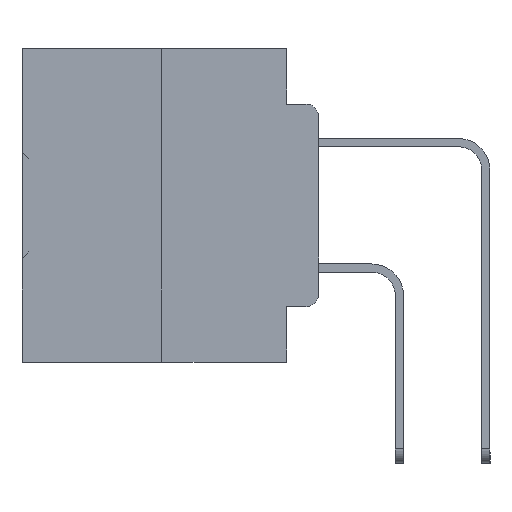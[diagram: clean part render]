
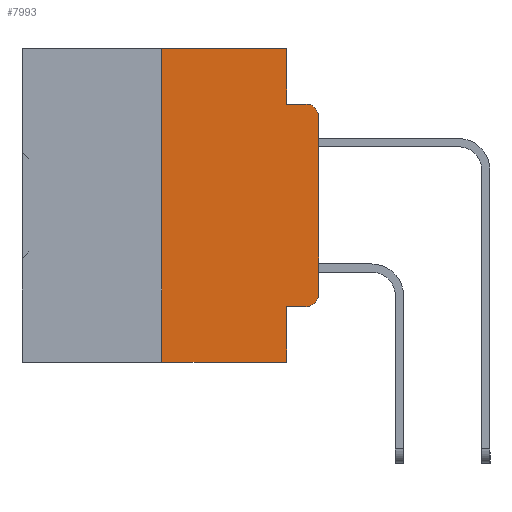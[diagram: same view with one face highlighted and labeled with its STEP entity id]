
A CAD part, left-side view. The second image highlights one B-rep face of the part: STEP entity #7993.
In plain terms, the highlighted planar face has unit normal (-1, 0, 0).
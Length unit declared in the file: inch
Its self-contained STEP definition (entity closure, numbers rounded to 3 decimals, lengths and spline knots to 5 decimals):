
#244 = EDGE_CURVE ( 'NONE', #16485, #21619, #24784, .T. ) ;
#370 = AXIS2_PLACEMENT_3D ( 'NONE', #22116, #3656, #25164 ) ;
#1568 = CARTESIAN_POINT ( 'NONE',  ( 0., 0.051, -0.4115 ) ) ;
#2293 = EDGE_CURVE ( 'NONE', #29441, #16485, #23737, .T. ) ;
#2381 = CARTESIAN_POINT ( 'NONE',  ( 0., 0.02, -0.0885 ) ) ;
#2928 = ORIENTED_EDGE ( 'NONE', *, *, #25778, .F. ) ;
#3067 = CARTESIAN_POINT ( 'NONE',  ( 0., 0.051, 0. ) ) ;
#3404 = ORIENTED_EDGE ( 'NONE', *, *, #37893, .F. ) ;
#3656 = DIRECTION ( 'NONE',  ( -1., 0., 0. ) ) ;
#4323 = ORIENTED_EDGE ( 'NONE', *, *, #13835, .T. ) ;
#5776 = CARTESIAN_POINT ( 'NONE',  ( 0., 0.473, 0. ) ) ;
#6856 = LINE ( 'NONE', #16288, #30311 ) ;
#6938 = CARTESIAN_POINT ( 'NONE',  ( 0., 0.051, -0.0885 ) ) ;
#7919 = CARTESIAN_POINT ( 'NONE',  ( 0., 0.473, 0. ) ) ;
#7993 = ADVANCED_FACE ( 'NONE', ( #14914 ), #30257, .F. ) ;
#8205 = VECTOR ( 'NONE', #10116, 39.37008 ) ;
#8875 = LINE ( 'NONE', #24295, #37418 ) ;
#8999 = DIRECTION ( 'NONE',  ( 0., -1., 0. ) ) ;
#9776 = EDGE_CURVE ( 'NONE', #32837, #11444, #29019, .T. ) ;
#10037 = LINE ( 'NONE', #13108, #33409 ) ;
#10041 = DIRECTION ( 'NONE',  ( 0., 0., -1. ) ) ;
#10116 = DIRECTION ( 'NONE',  ( 0., 0., -1. ) ) ;
#10364 = VERTEX_POINT ( 'NONE', #23327 ) ;
#10678 = CIRCLE ( 'NONE', #370, 0.02 ) ;
#10731 = CARTESIAN_POINT ( 'NONE',  ( 0., 0.02, -0.1085 ) ) ;
#11444 = VERTEX_POINT ( 'NONE', #3067 ) ;
#13108 = CARTESIAN_POINT ( 'NONE',  ( 0., 0.25, 0. ) ) ;
#13145 = ORIENTED_EDGE ( 'NONE', *, *, #17663, .T. ) ;
#13481 = DIRECTION ( 'NONE',  ( 0., 0., 1. ) ) ;
#13612 = ORIENTED_EDGE ( 'NONE', *, *, #9776, .F. ) ;
#13835 = EDGE_CURVE ( 'NONE', #10364, #39304, #8875, .T. ) ;
#13854 = LINE ( 'NONE', #16884, #38030 ) ;
#14914 = FACE_OUTER_BOUND ( 'NONE', #22867, .T. ) ;
#15589 = EDGE_CURVE ( 'NONE', #24892, #29441, #10678, .T. ) ;
#16228 = CARTESIAN_POINT ( 'NONE',  ( 0., 0.051, -0.4115 ) ) ;
#16288 = CARTESIAN_POINT ( 'NONE',  ( 0., 0.051, 0. ) ) ;
#16485 = VERTEX_POINT ( 'NONE', #23121 ) ;
#16884 = CARTESIAN_POINT ( 'NONE',  ( 0., 0.051, -0.0885 ) ) ;
#17663 = EDGE_CURVE ( 'NONE', #33151, #24892, #30477, .T. ) ;
#18224 = DIRECTION ( 'NONE',  ( 0., 0., -1. ) ) ;
#18932 = ORIENTED_EDGE ( 'NONE', *, *, #244, .T. ) ;
#20579 = CARTESIAN_POINT ( 'NONE',  ( 0., 0., -0.3915 ) ) ;
#20814 = ORIENTED_EDGE ( 'NONE', *, *, #29831, .F. ) ;
#20932 = CARTESIAN_POINT ( 'NONE',  ( 0., 0.051, -0.5 ) ) ;
#21330 = VERTEX_POINT ( 'NONE', #6938 ) ;
#21619 = VERTEX_POINT ( 'NONE', #2381 ) ;
#21739 = ORIENTED_EDGE ( 'NONE', *, *, #27785, .F. ) ;
#22116 = CARTESIAN_POINT ( 'NONE',  ( 0., 0.02, -0.3915 ) ) ;
#22867 = EDGE_LOOP ( 'NONE', ( #26009, #18932, #3404, #20814, #13612, #21739, #4323, #2928, #13145, #37335 ) ) ;
#22903 = VECTOR ( 'NONE', #29284, 39.37008 ) ;
#23121 = CARTESIAN_POINT ( 'NONE',  ( 0., 0., -0.1085 ) ) ;
#23327 = CARTESIAN_POINT ( 'NONE',  ( 0., 0.25, -0.5 ) ) ;
#23385 = VECTOR ( 'NONE', #37358, 39.37008 ) ;
#23723 = AXIS2_PLACEMENT_3D ( 'NONE', #5776, #36305, #18224 ) ;
#23737 = LINE ( 'NONE', #31703, #30823 ) ;
#24295 = CARTESIAN_POINT ( 'NONE',  ( 0., 0.473, -0.5 ) ) ;
#24784 = CIRCLE ( 'NONE', #30597, 0.02 ) ;
#24892 = VERTEX_POINT ( 'NONE', #27155 ) ;
#25164 = DIRECTION ( 'NONE',  ( 0., 0., -1. ) ) ;
#25706 = DIRECTION ( 'NONE',  ( 0., 0., -1. ) ) ;
#25778 = EDGE_CURVE ( 'NONE', #33151, #39304, #33520, .T. ) ;
#26009 = ORIENTED_EDGE ( 'NONE', *, *, #2293, .T. ) ;
#27155 = CARTESIAN_POINT ( 'NONE',  ( 0., 0.02, -0.4115 ) ) ;
#27785 = EDGE_CURVE ( 'NONE', #10364, #32837, #10037, .T. ) ;
#28595 = DIRECTION ( 'NONE',  ( -1., 0., 0. ) ) ;
#29019 = LINE ( 'NONE', #7919, #22903 ) ;
#29167 = CARTESIAN_POINT ( 'NONE',  ( 0., 0.25, 0. ) ) ;
#29284 = DIRECTION ( 'NONE',  ( 0., -1., 0. ) ) ;
#29441 = VERTEX_POINT ( 'NONE', #20579 ) ;
#29831 = EDGE_CURVE ( 'NONE', #11444, #21330, #6856, .T. ) ;
#30257 = PLANE ( 'NONE',  #23723 ) ;
#30311 = VECTOR ( 'NONE', #10041, 39.37008 ) ;
#30477 = LINE ( 'NONE', #16228, #23385 ) ;
#30597 = AXIS2_PLACEMENT_3D ( 'NONE', #10731, #28595, #25706 ) ;
#30823 = VECTOR ( 'NONE', #13481, 39.37008 ) ;
#31459 = CARTESIAN_POINT ( 'NONE',  ( 0., 0.051, 0. ) ) ;
#31703 = CARTESIAN_POINT ( 'NONE',  ( 0., 0., 0. ) ) ;
#32837 = VERTEX_POINT ( 'NONE', #29167 ) ;
#33151 = VERTEX_POINT ( 'NONE', #1568 ) ;
#33409 = VECTOR ( 'NONE', #37364, 39.37008 ) ;
#33520 = LINE ( 'NONE', #31459, #8205 ) ;
#35033 = DIRECTION ( 'NONE',  ( 0., -1., 0. ) ) ;
#36305 = DIRECTION ( 'NONE',  ( 1., 0., 0. ) ) ;
#37335 = ORIENTED_EDGE ( 'NONE', *, *, #15589, .T. ) ;
#37358 = DIRECTION ( 'NONE',  ( 0., -1., 0. ) ) ;
#37364 = DIRECTION ( 'NONE',  ( 0., 0., 1. ) ) ;
#37418 = VECTOR ( 'NONE', #8999, 39.37008 ) ;
#37893 = EDGE_CURVE ( 'NONE', #21330, #21619, #13854, .T. ) ;
#38030 = VECTOR ( 'NONE', #35033, 39.37008 ) ;
#39304 = VERTEX_POINT ( 'NONE', #20932 ) ;
